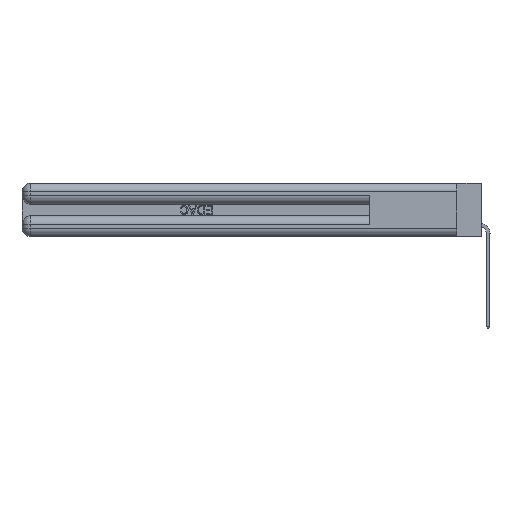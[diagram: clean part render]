
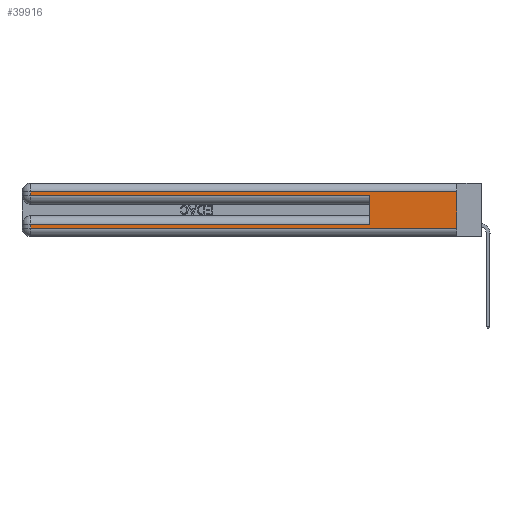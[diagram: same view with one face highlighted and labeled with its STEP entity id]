
A CAD part, left-side view. The second image highlights one B-rep face of the part: STEP entity #39916.
In plain terms, the highlighted planar face has unit normal (-1, 0, 0).
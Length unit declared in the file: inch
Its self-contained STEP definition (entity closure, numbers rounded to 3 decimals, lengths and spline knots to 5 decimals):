
#2558 = LINE ( 'NONE', #24188, #40891 ) ;
#2646 = EDGE_CURVE ( 'NONE', #36116, #39411, #2558, .T. ) ;
#3681 = EDGE_CURVE ( 'NONE', #9042, #39683, #4180, .T. ) ;
#4180 = LINE ( 'NONE', #12228, #27505 ) ;
#5912 = LINE ( 'NONE', #42461, #13453 ) ;
#7220 = ORIENTED_EDGE ( 'NONE', *, *, #40962, .T. ) ;
#7547 = PLANE ( 'NONE',  #36238 ) ;
#7839 = DIRECTION ( 'NONE',  ( 0., 1., 0. ) ) ;
#8046 = ORIENTED_EDGE ( 'NONE', *, *, #19732, .T. ) ;
#9042 = VERTEX_POINT ( 'NONE', #38448 ) ;
#10221 = CARTESIAN_POINT ( 'NONE',  ( 0., 0.6, 0.085 ) ) ;
#10493 = CARTESIAN_POINT ( 'NONE',  ( 0., 0., 0.31 ) ) ;
#11099 = DIRECTION ( 'NONE',  ( 0., 0., -1. ) ) ;
#12228 = CARTESIAN_POINT ( 'NONE',  ( 0., 0., 0.285 ) ) ;
#12572 = VERTEX_POINT ( 'NONE', #43266 ) ;
#12888 = DIRECTION ( 'NONE',  ( 0., 0., 1. ) ) ;
#13453 = VECTOR ( 'NONE', #12888, 39.37008 ) ;
#13999 = VECTOR ( 'NONE', #26541, 39.37008 ) ;
#15313 = ORIENTED_EDGE ( 'NONE', *, *, #39314, .F. ) ;
#16161 = CARTESIAN_POINT ( 'NONE',  ( 0., 0., 0.06 ) ) ;
#18037 = CARTESIAN_POINT ( 'NONE',  ( 0., 0., 0.37 ) ) ;
#18298 = ORIENTED_EDGE ( 'NONE', *, *, #21280, .F. ) ;
#18904 = CARTESIAN_POINT ( 'NONE',  ( 0., 2.94, 0.085 ) ) ;
#19732 = EDGE_CURVE ( 'NONE', #39411, #41157, #22857, .T. ) ;
#20163 = ORIENTED_EDGE ( 'NONE', *, *, #23608, .T. ) ;
#20183 = VECTOR ( 'NONE', #35527, 39.37008 ) ;
#20624 = FACE_OUTER_BOUND ( 'NONE', #38665, .T. ) ;
#21280 = EDGE_CURVE ( 'NONE', #36116, #39683, #5912, .T. ) ;
#21751 = VECTOR ( 'NONE', #45774, 39.37008 ) ;
#22466 = CARTESIAN_POINT ( 'NONE',  ( 0., 0., 0.37 ) ) ;
#22471 = VECTOR ( 'NONE', #31891, 39.37008 ) ;
#22857 = LINE ( 'NONE', #33181, #21751 ) ;
#23608 = EDGE_CURVE ( 'NONE', #12572, #9042, #38158, .T. ) ;
#23849 = DIRECTION ( 'NONE',  ( 0., 1., 0. ) ) ;
#24188 = CARTESIAN_POINT ( 'NONE',  ( 0., 0., 0.085 ) ) ;
#24663 = VECTOR ( 'NONE', #7839, 39.37008 ) ;
#25200 = CARTESIAN_POINT ( 'NONE',  ( 0., 0., 0.06 ) ) ;
#26541 = DIRECTION ( 'NONE',  ( 0., 0., -1. ) ) ;
#27232 = DIRECTION ( 'NONE',  ( 0., -1., 0. ) ) ;
#27505 = VECTOR ( 'NONE', #27232, 39.37008 ) ;
#29431 = CARTESIAN_POINT ( 'NONE',  ( 0., 0.6, 0.285 ) ) ;
#30515 = EDGE_CURVE ( 'NONE', #35792, #12572, #47912, .T. ) ;
#31891 = DIRECTION ( 'NONE',  ( 0., -1., 0. ) ) ;
#32329 = CARTESIAN_POINT ( 'NONE',  ( 0., 2.94, 0.37 ) ) ;
#33181 = CARTESIAN_POINT ( 'NONE',  ( 0., 2.94, 0.37 ) ) ;
#33573 = DIRECTION ( 'NONE',  ( 1., 0., 0. ) ) ;
#34726 = VERTEX_POINT ( 'NONE', #16161 ) ;
#35527 = DIRECTION ( 'NONE',  ( 0., 0., -1. ) ) ;
#35792 = VERTEX_POINT ( 'NONE', #40922 ) ;
#36116 = VERTEX_POINT ( 'NONE', #10221 ) ;
#36238 = AXIS2_PLACEMENT_3D ( 'NONE', #22466, #33573, #11099 ) ;
#37580 = LINE ( 'NONE', #25200, #22471 ) ;
#38158 = LINE ( 'NONE', #32329, #20183 ) ;
#38448 = CARTESIAN_POINT ( 'NONE',  ( 0., 2.94, 0.285 ) ) ;
#38665 = EDGE_LOOP ( 'NONE', ( #15313, #42480, #20163, #41297, #18298, #41668, #8046, #7220 ) ) ;
#39314 = EDGE_CURVE ( 'NONE', #35792, #34726, #45308, .T. ) ;
#39411 = VERTEX_POINT ( 'NONE', #18904 ) ;
#39683 = VERTEX_POINT ( 'NONE', #29431 ) ;
#39916 = ADVANCED_FACE ( 'NONE', ( #20624 ), #7547, .F. ) ;
#40880 = CARTESIAN_POINT ( 'NONE',  ( 0., 2.94, 0.06 ) ) ;
#40891 = VECTOR ( 'NONE', #23849, 39.37008 ) ;
#40922 = CARTESIAN_POINT ( 'NONE',  ( 0., 0., 0.31 ) ) ;
#40962 = EDGE_CURVE ( 'NONE', #41157, #34726, #37580, .T. ) ;
#41157 = VERTEX_POINT ( 'NONE', #40880 ) ;
#41297 = ORIENTED_EDGE ( 'NONE', *, *, #3681, .T. ) ;
#41668 = ORIENTED_EDGE ( 'NONE', *, *, #2646, .T. ) ;
#42461 = CARTESIAN_POINT ( 'NONE',  ( 0., 0.6, 0.145 ) ) ;
#42480 = ORIENTED_EDGE ( 'NONE', *, *, #30515, .T. ) ;
#43266 = CARTESIAN_POINT ( 'NONE',  ( 0., 2.94, 0.31 ) ) ;
#45308 = LINE ( 'NONE', #18037, #13999 ) ;
#45774 = DIRECTION ( 'NONE',  ( 0., 0., -1. ) ) ;
#47912 = LINE ( 'NONE', #10493, #24663 ) ;
